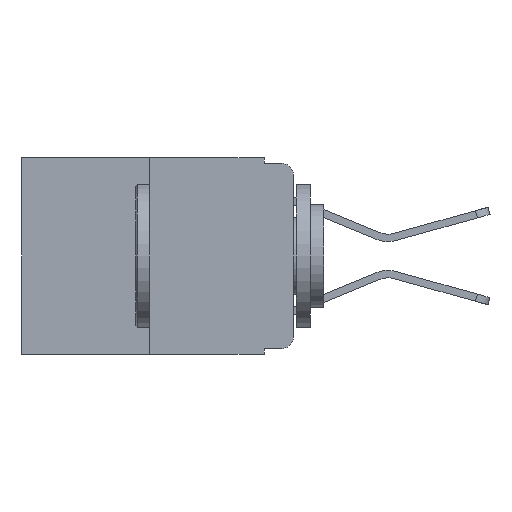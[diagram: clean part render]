
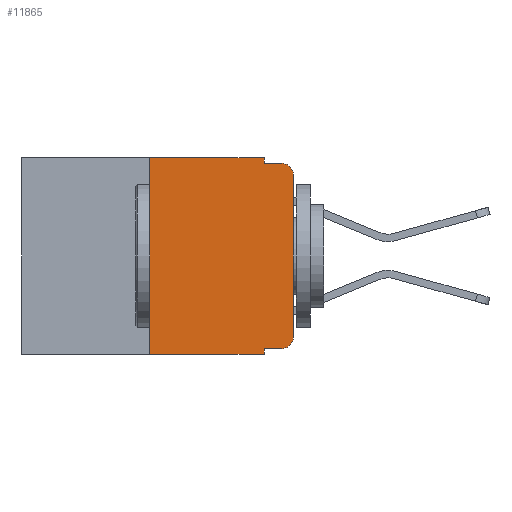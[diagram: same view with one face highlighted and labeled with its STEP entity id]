
A CAD part, left-side view. The second image highlights one B-rep face of the part: STEP entity #11865.
In plain terms, the highlighted planar face has unit normal (-1, 0, 0).
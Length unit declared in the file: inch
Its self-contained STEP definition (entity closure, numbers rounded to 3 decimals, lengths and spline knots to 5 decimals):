
#61 = DIRECTION ( 'NONE',  ( 0., -1., 0. ) ) ;
#307 = AXIS2_PLACEMENT_3D ( 'NONE', #17847, #17807, #13639 ) ;
#632 = LINE ( 'NONE', #10861, #8413 ) ;
#702 = VERTEX_POINT ( 'NONE', #4866 ) ;
#810 = DIRECTION ( 'NONE',  ( 0., 0., -1. ) ) ;
#2220 = EDGE_CURVE ( 'NONE', #12759, #14671, #6814, .T. ) ;
#2348 = CARTESIAN_POINT ( 'NONE',  ( 0., 0.051, -0.01 ) ) ;
#2651 = CIRCLE ( 'NONE', #16203, 0.02 ) ;
#2657 = VECTOR ( 'NONE', #15446, 39.37008 ) ;
#2901 = DIRECTION ( 'NONE',  ( 0., -1., 0. ) ) ;
#2905 = EDGE_CURVE ( 'NONE', #17525, #702, #6932, .T. ) ;
#3765 = LINE ( 'NONE', #8542, #7848 ) ;
#4251 = DIRECTION ( 'NONE',  ( 1., 0., 0. ) ) ;
#4440 = CARTESIAN_POINT ( 'NONE',  ( 0., 0.051, -0.333 ) ) ;
#4866 = CARTESIAN_POINT ( 'NONE',  ( 0., 0., -0.03 ) ) ;
#4977 = ORIENTED_EDGE ( 'NONE', *, *, #17859, .F. ) ;
#5107 = CARTESIAN_POINT ( 'NONE',  ( 0., 0.25, -0.343 ) ) ;
#5314 = DIRECTION ( 'NONE',  ( 0., 0., -1. ) ) ;
#5342 = VECTOR ( 'NONE', #5994, 39.37008 ) ;
#5376 = EDGE_CURVE ( 'NONE', #702, #18209, #7809, .T. ) ;
#5432 = EDGE_CURVE ( 'NONE', #14671, #6092, #14393, .T. ) ;
#5994 = DIRECTION ( 'NONE',  ( 0., -1., 0. ) ) ;
#6092 = VERTEX_POINT ( 'NONE', #9701 ) ;
#6169 = VECTOR ( 'NONE', #8867, 39.37008 ) ;
#6697 = VECTOR ( 'NONE', #11533, 39.37008 ) ;
#6807 = EDGE_CURVE ( 'NONE', #10380, #17525, #2651, .T. ) ;
#6814 = LINE ( 'NONE', #7507, #2657 ) ;
#6932 = LINE ( 'NONE', #12263, #18408 ) ;
#7507 = CARTESIAN_POINT ( 'NONE',  ( 0., 0.25, 0. ) ) ;
#7809 = CIRCLE ( 'NONE', #307, 0.02 ) ;
#7848 = VECTOR ( 'NONE', #810, 39.37008 ) ;
#8208 = EDGE_CURVE ( 'NONE', #12759, #12604, #632, .T. ) ;
#8413 = VECTOR ( 'NONE', #61, 39.37008 ) ;
#8542 = CARTESIAN_POINT ( 'NONE',  ( 0., 0.051, 0. ) ) ;
#8606 = CARTESIAN_POINT ( 'NONE',  ( 0., 0.051, -0.343 ) ) ;
#8867 = DIRECTION ( 'NONE',  ( 0., 0., -1. ) ) ;
#9003 = ORIENTED_EDGE ( 'NONE', *, *, #5376, .T. ) ;
#9421 = LINE ( 'NONE', #4440, #5342 ) ;
#9495 = ORIENTED_EDGE ( 'NONE', *, *, #10463, .F. ) ;
#9701 = CARTESIAN_POINT ( 'NONE',  ( 0., 0.051, 0. ) ) ;
#9774 = EDGE_LOOP ( 'NONE', ( #17615, #9003, #9495, #4977, #18157, #12117, #17017, #14920, #19334, #13776 ) ) ;
#9899 = VERTEX_POINT ( 'NONE', #11950 ) ;
#10380 = VERTEX_POINT ( 'NONE', #15791 ) ;
#10399 = VECTOR ( 'NONE', #2901, 39.37008 ) ;
#10402 = DIRECTION ( 'NONE',  ( 0., 0., 1. ) ) ;
#10463 = EDGE_CURVE ( 'NONE', #13987, #18209, #10694, .T. ) ;
#10694 = LINE ( 'NONE', #2348, #6697 ) ;
#10861 = CARTESIAN_POINT ( 'NONE',  ( 0., 0.473, -0.343 ) ) ;
#10994 = DIRECTION ( 'NONE',  ( -1., 0., 0. ) ) ;
#11533 = DIRECTION ( 'NONE',  ( 0., -1., 0. ) ) ;
#11832 = CARTESIAN_POINT ( 'NONE',  ( 0., 0.473, 0. ) ) ;
#11865 = ADVANCED_FACE ( 'NONE', ( #14183 ), #13346, .F. ) ;
#11876 = EDGE_CURVE ( 'NONE', #9899, #12604, #18577, .T. ) ;
#11950 = CARTESIAN_POINT ( 'NONE',  ( 0., 0.051, -0.333 ) ) ;
#12117 = ORIENTED_EDGE ( 'NONE', *, *, #2220, .F. ) ;
#12217 = CARTESIAN_POINT ( 'NONE',  ( 0., 0.051, -0.01 ) ) ;
#12263 = CARTESIAN_POINT ( 'NONE',  ( 0., 0., 0. ) ) ;
#12604 = VERTEX_POINT ( 'NONE', #8606 ) ;
#12759 = VERTEX_POINT ( 'NONE', #5107 ) ;
#13029 = CARTESIAN_POINT ( 'NONE',  ( 0., 0.02, -0.313 ) ) ;
#13346 = PLANE ( 'NONE',  #17517 ) ;
#13639 = DIRECTION ( 'NONE',  ( 0., 0., -1. ) ) ;
#13776 = ORIENTED_EDGE ( 'NONE', *, *, #6807, .T. ) ;
#13898 = EDGE_CURVE ( 'NONE', #9899, #10380, #9421, .T. ) ;
#13987 = VERTEX_POINT ( 'NONE', #12217 ) ;
#14183 = FACE_OUTER_BOUND ( 'NONE', #9774, .T. ) ;
#14393 = LINE ( 'NONE', #18814, #10399 ) ;
#14671 = VERTEX_POINT ( 'NONE', #18504 ) ;
#14833 = DIRECTION ( 'NONE',  ( 0., 0., -1. ) ) ;
#14920 = ORIENTED_EDGE ( 'NONE', *, *, #11876, .F. ) ;
#15427 = CARTESIAN_POINT ( 'NONE',  ( 0., 0.02, -0.01 ) ) ;
#15446 = DIRECTION ( 'NONE',  ( 0., 0., 1. ) ) ;
#15791 = CARTESIAN_POINT ( 'NONE',  ( 0., 0.02, -0.333 ) ) ;
#16203 = AXIS2_PLACEMENT_3D ( 'NONE', #13029, #10994, #5314 ) ;
#16448 = CARTESIAN_POINT ( 'NONE',  ( 0., 0., -0.313 ) ) ;
#17017 = ORIENTED_EDGE ( 'NONE', *, *, #8208, .T. ) ;
#17517 = AXIS2_PLACEMENT_3D ( 'NONE', #11832, #4251, #14833 ) ;
#17525 = VERTEX_POINT ( 'NONE', #16448 ) ;
#17615 = ORIENTED_EDGE ( 'NONE', *, *, #2905, .T. ) ;
#17807 = DIRECTION ( 'NONE',  ( -1., 0., 0. ) ) ;
#17847 = CARTESIAN_POINT ( 'NONE',  ( 0., 0.02, -0.03 ) ) ;
#17859 = EDGE_CURVE ( 'NONE', #6092, #13987, #3765, .T. ) ;
#18157 = ORIENTED_EDGE ( 'NONE', *, *, #5432, .F. ) ;
#18209 = VERTEX_POINT ( 'NONE', #15427 ) ;
#18408 = VECTOR ( 'NONE', #10402, 39.37008 ) ;
#18504 = CARTESIAN_POINT ( 'NONE',  ( 0., 0.25, 0. ) ) ;
#18577 = LINE ( 'NONE', #19243, #6169 ) ;
#18814 = CARTESIAN_POINT ( 'NONE',  ( 0., 0.473, 0. ) ) ;
#19243 = CARTESIAN_POINT ( 'NONE',  ( 0., 0.051, 0. ) ) ;
#19334 = ORIENTED_EDGE ( 'NONE', *, *, #13898, .T. ) ;
